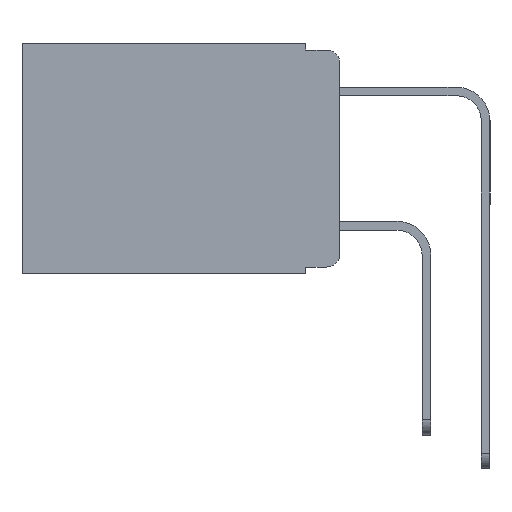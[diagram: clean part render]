
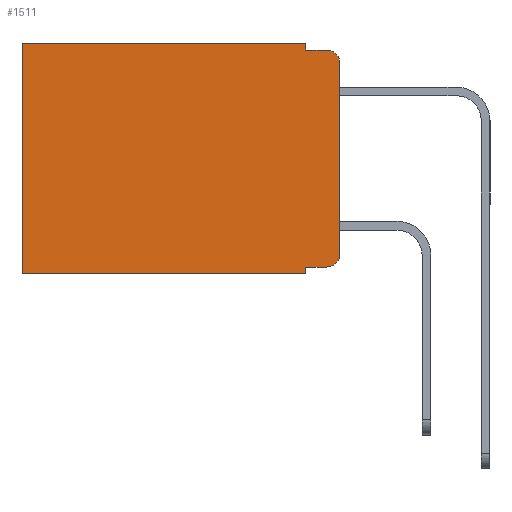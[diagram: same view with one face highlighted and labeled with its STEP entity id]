
A CAD part, left-side view. The second image highlights one B-rep face of the part: STEP entity #1511.
In plain terms, the highlighted planar face has unit normal (-1, 0, 0).
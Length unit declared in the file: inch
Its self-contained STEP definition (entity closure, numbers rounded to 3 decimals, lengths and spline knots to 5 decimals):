
#227 = VECTOR ( 'NONE', #14607, 39.37008 ) ;
#382 = DIRECTION ( 'NONE',  ( 0., 0., -1. ) ) ;
#695 = EDGE_CURVE ( 'NONE', #16299, #10997, #3078, .T. ) ;
#1511 = ADVANCED_FACE ( 'NONE', ( #15886 ), #5183, .F. ) ;
#1949 = ORIENTED_EDGE ( 'NONE', *, *, #6975, .T. ) ;
#2090 = LINE ( 'NONE', #8027, #9629 ) ;
#2972 = ORIENTED_EDGE ( 'NONE', *, *, #6447, .T. ) ;
#3078 = CIRCLE ( 'NONE', #16145, 0.02 ) ;
#3286 = DIRECTION ( 'NONE',  ( 0., 1., 0. ) ) ;
#3587 = VERTEX_POINT ( 'NONE', #8466 ) ;
#3626 = LINE ( 'NONE', #16199, #7723 ) ;
#3666 = AXIS2_PLACEMENT_3D ( 'NONE', #6394, #15805, #7970 ) ;
#3693 = CARTESIAN_POINT ( 'NONE',  ( 0.298, 0.051, -0.333 ) ) ;
#3931 = DIRECTION ( 'NONE',  ( 0., 0., -1. ) ) ;
#4108 = VERTEX_POINT ( 'NONE', #6522 ) ;
#4207 = AXIS2_PLACEMENT_3D ( 'NONE', #12481, #5100, #12531 ) ;
#4320 = CARTESIAN_POINT ( 'NONE',  ( 0.298, 0.02, -0.01 ) ) ;
#4607 = VECTOR ( 'NONE', #8281, 39.37008 ) ;
#5078 = LINE ( 'NONE', #10920, #227 ) ;
#5100 = DIRECTION ( 'NONE',  ( 1., 0., 0. ) ) ;
#5183 = PLANE ( 'NONE',  #4207 ) ;
#5431 = VERTEX_POINT ( 'NONE', #6464 ) ;
#6286 = VERTEX_POINT ( 'NONE', #10183 ) ;
#6355 = ORIENTED_EDGE ( 'NONE', *, *, #695, .T. ) ;
#6394 = CARTESIAN_POINT ( 'NONE',  ( 0.298, 0.02, -0.313 ) ) ;
#6447 = EDGE_CURVE ( 'NONE', #5431, #3587, #15598, .T. ) ;
#6462 = CARTESIAN_POINT ( 'NONE',  ( 0.298, 0.051, 0. ) ) ;
#6464 = CARTESIAN_POINT ( 'NONE',  ( 0.298, 0.051, 0. ) ) ;
#6522 = CARTESIAN_POINT ( 'NONE',  ( 0.298, 0.473, -0.343 ) ) ;
#6826 = ORIENTED_EDGE ( 'NONE', *, *, #7035, .F. ) ;
#6942 = EDGE_CURVE ( 'NONE', #6286, #14979, #9022, .T. ) ;
#6968 = EDGE_CURVE ( 'NONE', #17307, #6286, #5078, .T. ) ;
#6972 = EDGE_CURVE ( 'NONE', #17307, #12688, #15543, .T. ) ;
#6975 = EDGE_CURVE ( 'NONE', #3587, #4108, #15176, .T. ) ;
#7002 = EDGE_CURVE ( 'NONE', #5431, #14959, #3626, .T. ) ;
#7006 = EDGE_CURVE ( 'NONE', #14959, #10997, #14355, .T. ) ;
#7035 = EDGE_CURVE ( 'NONE', #16299, #14979, #17301, .T. ) ;
#7117 = CARTESIAN_POINT ( 'NONE',  ( 0.298, 0., -0.03 ) ) ;
#7210 = VECTOR ( 'NONE', #11066, 39.37008 ) ;
#7338 = EDGE_CURVE ( 'NONE', #12688, #4108, #2090, .T. ) ;
#7723 = VECTOR ( 'NONE', #17431, 39.37008 ) ;
#7970 = DIRECTION ( 'NONE',  ( 0., 0., -1. ) ) ;
#8027 = CARTESIAN_POINT ( 'NONE',  ( 0.298, 0., -0.343 ) ) ;
#8190 = VECTOR ( 'NONE', #382, 39.37008 ) ;
#8281 = DIRECTION ( 'NONE',  ( 0., 0., -1. ) ) ;
#8282 = DIRECTION ( 'NONE',  ( 0., 0., -1. ) ) ;
#8291 = CARTESIAN_POINT ( 'NONE',  ( 0.298, 0.051, -0.01 ) ) ;
#8466 = CARTESIAN_POINT ( 'NONE',  ( 0.298, 0.473, 0. ) ) ;
#9022 = CIRCLE ( 'NONE', #3666, 0.02 ) ;
#9629 = VECTOR ( 'NONE', #3286, 39.37008 ) ;
#9734 = CARTESIAN_POINT ( 'NONE',  ( 0.298, 0.051, -0.01 ) ) ;
#10076 = VECTOR ( 'NONE', #3931, 39.37008 ) ;
#10183 = CARTESIAN_POINT ( 'NONE',  ( 0.298, 0.02, -0.333 ) ) ;
#10579 = ORIENTED_EDGE ( 'NONE', *, *, #7002, .F. ) ;
#10634 = DIRECTION ( 'NONE',  ( 0., 1., 0. ) ) ;
#10779 = ORIENTED_EDGE ( 'NONE', *, *, #6972, .F. ) ;
#10875 = EDGE_LOOP ( 'NONE', ( #6826, #6355, #17770, #10579, #2972, #1949, #14235, #10779, #15055, #11182 ) ) ;
#10920 = CARTESIAN_POINT ( 'NONE',  ( 0.298, 0.051, -0.333 ) ) ;
#10997 = VERTEX_POINT ( 'NONE', #4320 ) ;
#11066 = DIRECTION ( 'NONE',  ( 0., -1., 0. ) ) ;
#11123 = CARTESIAN_POINT ( 'NONE',  ( 0.298, 0., 0. ) ) ;
#11182 = ORIENTED_EDGE ( 'NONE', *, *, #6942, .T. ) ;
#11354 = CARTESIAN_POINT ( 'NONE',  ( 0.298, 0.02, -0.03 ) ) ;
#12481 = CARTESIAN_POINT ( 'NONE',  ( 0.298, 0., 0. ) ) ;
#12531 = DIRECTION ( 'NONE',  ( 0., 0., -1. ) ) ;
#12688 = VERTEX_POINT ( 'NONE', #12982 ) ;
#12982 = CARTESIAN_POINT ( 'NONE',  ( 0.298, 0.051, -0.343 ) ) ;
#13719 = DIRECTION ( 'NONE',  ( -1., 0., 0. ) ) ;
#14235 = ORIENTED_EDGE ( 'NONE', *, *, #7338, .F. ) ;
#14355 = LINE ( 'NONE', #9734, #7210 ) ;
#14607 = DIRECTION ( 'NONE',  ( 0., -1., 0. ) ) ;
#14956 = CARTESIAN_POINT ( 'NONE',  ( 0.298, 0., -0.313 ) ) ;
#14959 = VERTEX_POINT ( 'NONE', #8291 ) ;
#14979 = VERTEX_POINT ( 'NONE', #14956 ) ;
#15055 = ORIENTED_EDGE ( 'NONE', *, *, #6968, .T. ) ;
#15176 = LINE ( 'NONE', #17331, #8190 ) ;
#15543 = LINE ( 'NONE', #6462, #4607 ) ;
#15598 = LINE ( 'NONE', #17027, #18139 ) ;
#15805 = DIRECTION ( 'NONE',  ( -1., 0., 0. ) ) ;
#15886 = FACE_OUTER_BOUND ( 'NONE', #10875, .T. ) ;
#16145 = AXIS2_PLACEMENT_3D ( 'NONE', #11354, #13719, #8282 ) ;
#16199 = CARTESIAN_POINT ( 'NONE',  ( 0.298, 0.051, 0. ) ) ;
#16299 = VERTEX_POINT ( 'NONE', #7117 ) ;
#17027 = CARTESIAN_POINT ( 'NONE',  ( 0.298, 0., 0. ) ) ;
#17301 = LINE ( 'NONE', #11123, #10076 ) ;
#17307 = VERTEX_POINT ( 'NONE', #3693 ) ;
#17331 = CARTESIAN_POINT ( 'NONE',  ( 0.298, 0.473, 0. ) ) ;
#17431 = DIRECTION ( 'NONE',  ( 0., 0., -1. ) ) ;
#17770 = ORIENTED_EDGE ( 'NONE', *, *, #7006, .F. ) ;
#18139 = VECTOR ( 'NONE', #10634, 39.37008 ) ;
